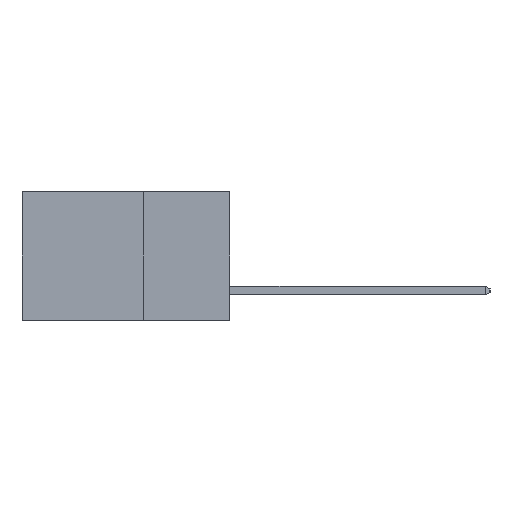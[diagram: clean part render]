
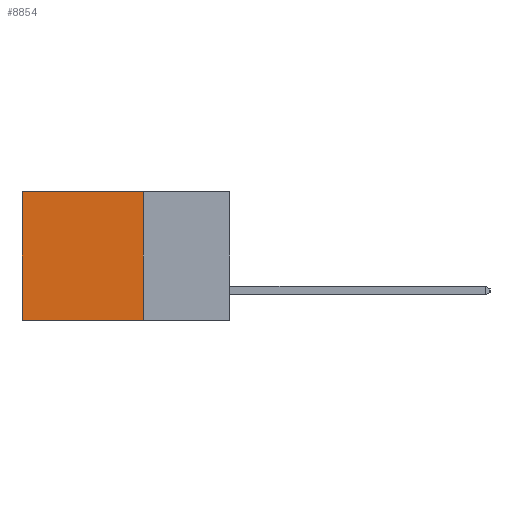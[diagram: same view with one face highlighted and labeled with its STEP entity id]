
A CAD part, left-side view. The second image highlights one B-rep face of the part: STEP entity #8854.
In plain terms, the highlighted planar face has unit normal (-1, 0, 0).
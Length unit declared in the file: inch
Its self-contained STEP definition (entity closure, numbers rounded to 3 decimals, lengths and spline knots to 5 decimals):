
#1154 = CARTESIAN_POINT ( 'NONE',  ( 0.298, 0.25, 0. ) ) ;
#1524 = CARTESIAN_POINT ( 'NONE',  ( 0.298, 0.25, -0.37 ) ) ;
#1567 = CARTESIAN_POINT ( 'NONE',  ( 0.298, 0.25, -0.37 ) ) ;
#1662 = DIRECTION ( 'NONE',  ( 0., 1., 0. ) ) ;
#1700 = LINE ( 'NONE', #1567, #20748 ) ;
#1762 = CARTESIAN_POINT ( 'NONE',  ( 0.298, 0.25, 0. ) ) ;
#2519 = VERTEX_POINT ( 'NONE', #1524 ) ;
#2737 = CARTESIAN_POINT ( 'NONE',  ( 0.298, 0.6, 0. ) ) ;
#3416 = AXIS2_PLACEMENT_3D ( 'NONE', #24922, #24900, #24866 ) ;
#3796 = DIRECTION ( 'NONE',  ( 0., 1., 0. ) ) ;
#3845 = CARTESIAN_POINT ( 'NONE',  ( 0.298, 0.25, 0. ) ) ;
#5320 = ORIENTED_EDGE ( 'NONE', *, *, #18978, .F. ) ;
#6872 = EDGE_CURVE ( 'NONE', #17983, #11240, #19358, .T. ) ;
#7597 = LINE ( 'NONE', #1154, #22425 ) ;
#8390 = VECTOR ( 'NONE', #3796, 39.37008 ) ;
#8814 = CARTESIAN_POINT ( 'NONE',  ( 0.298, 0.6, 0. ) ) ;
#8854 = ADVANCED_FACE ( 'NONE', ( #23086 ), #25495, .F. ) ;
#10746 = DIRECTION ( 'NONE',  ( 0., 0., -1. ) ) ;
#11240 = VERTEX_POINT ( 'NONE', #2737 ) ;
#13634 = CARTESIAN_POINT ( 'NONE',  ( 0.298, 0.6, -0.37 ) ) ;
#15196 = EDGE_CURVE ( 'NONE', #17983, #2519, #7597, .T. ) ;
#17983 = VERTEX_POINT ( 'NONE', #1762 ) ;
#18252 = EDGE_CURVE ( 'NONE', #11240, #22181, #24715, .T. ) ;
#18471 = VECTOR ( 'NONE', #10746, 39.37008 ) ;
#18978 = EDGE_CURVE ( 'NONE', #2519, #22181, #1700, .T. ) ;
#19358 = LINE ( 'NONE', #3845, #8390 ) ;
#20748 = VECTOR ( 'NONE', #1662, 39.37008 ) ;
#22181 = VERTEX_POINT ( 'NONE', #13634 ) ;
#22425 = VECTOR ( 'NONE', #24750, 39.37008 ) ;
#23086 = FACE_OUTER_BOUND ( 'NONE', #24902, .T. ) ;
#23451 = ORIENTED_EDGE ( 'NONE', *, *, #15196, .F. ) ;
#24129 = ORIENTED_EDGE ( 'NONE', *, *, #6872, .T. ) ;
#24715 = LINE ( 'NONE', #8814, #18471 ) ;
#24750 = DIRECTION ( 'NONE',  ( 0., 0., -1. ) ) ;
#24817 = ORIENTED_EDGE ( 'NONE', *, *, #18252, .T. ) ;
#24866 = DIRECTION ( 'NONE',  ( 0., 0., -1. ) ) ;
#24900 = DIRECTION ( 'NONE',  ( 1., 0., 0. ) ) ;
#24902 = EDGE_LOOP ( 'NONE', ( #24817, #5320, #23451, #24129 ) ) ;
#24922 = CARTESIAN_POINT ( 'NONE',  ( 0.298, 0.25, 0. ) ) ;
#25495 = PLANE ( 'NONE',  #3416 ) ;
